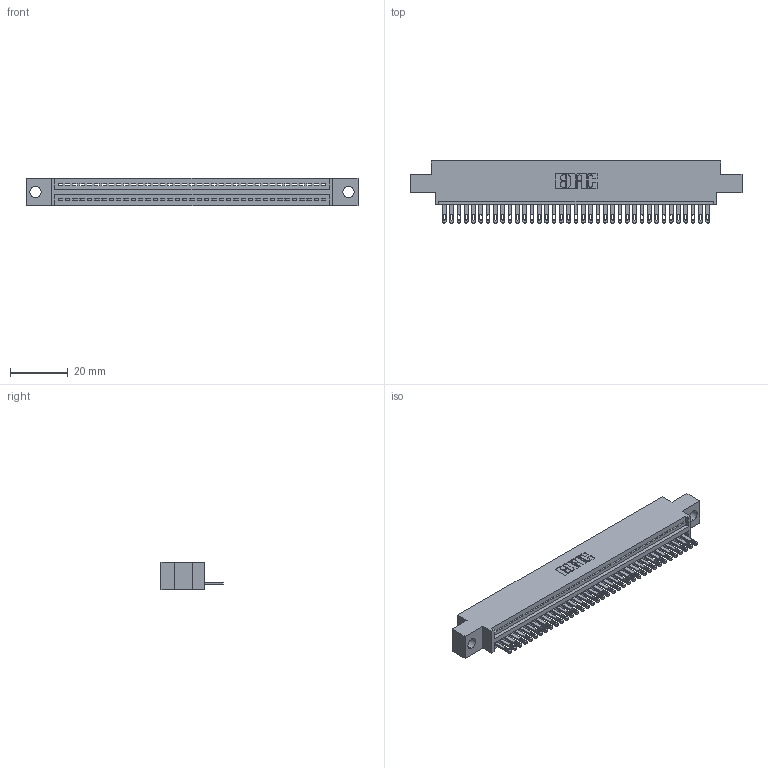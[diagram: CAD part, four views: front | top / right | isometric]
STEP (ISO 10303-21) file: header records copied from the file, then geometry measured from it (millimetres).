
FILE_DESCRIPTION (( 'STEP AP203' ), '1' );
FILE_NAME ('895-037-500-604.STEP', '2020-09-26T00:19:36', ( '' ), ( '' ), 'SwSTEP 2.0', 'SolidWorks 2020', '' );
FILE_SCHEMA (( 'CONFIG_CONTROL_DESIGN' ));
Length unit declared in the file: inch
Products named in the file (3): 845 Part_0.170 Offset - 0.156 Dia-TH; 345-292-001_345-293-100; 895-037-500-604
Assembly tree (38 placements, depth 2):
  895-037-500-604
    845 Part_0.170 Offset - 0.156 Dia-TH
    345-292-001_345-293-100  x37
Bounding box: 115.19 x 21.51 x 9.4 mm (x, y, z)
Volume: 10721.5 mm3; surface area: 14198.3 mm2
Topology: 38 solids, 38 shells, 2128 faces, 6569 edges, 4378 vertices
Faces by surface type: plane 1342, cylinder 786
Entity records: 28585 total; most frequent: CARTESIAN_POINT 4959, ORIENTED_EDGE 4930, DIRECTION 4339, EDGE_CURVE 2465, LINE 2181, VECTOR 2181, VERTEX_POINT 1642, AXIS2_PLACEMENT_3D 1079
